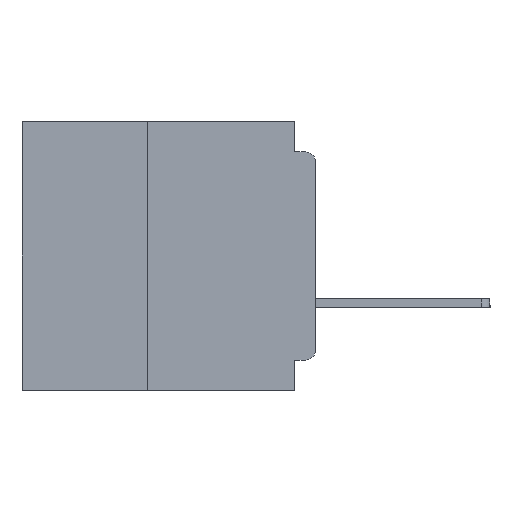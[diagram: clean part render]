
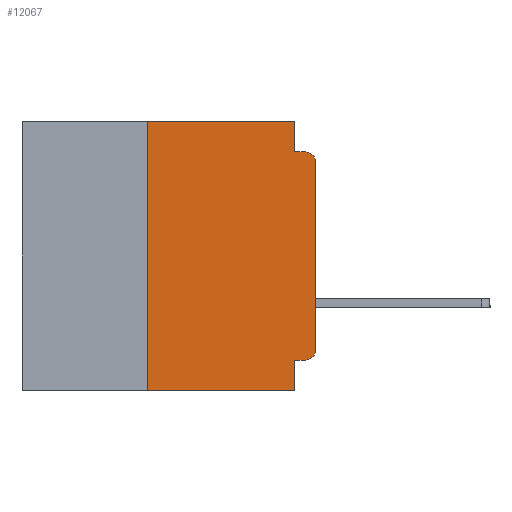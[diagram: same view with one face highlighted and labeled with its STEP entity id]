
A CAD part, left-side view. The second image highlights one B-rep face of the part: STEP entity #12067.
In plain terms, the highlighted planar face has unit normal (-1, 0, 0).
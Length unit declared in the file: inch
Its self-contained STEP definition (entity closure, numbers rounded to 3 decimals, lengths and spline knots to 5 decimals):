
#602 = ORIENTED_EDGE ( 'NONE', *, *, #23566, .F. ) ;
#1863 = DIRECTION ( 'NONE',  ( 0., 0., -1. ) ) ;
#2235 = CARTESIAN_POINT ( 'NONE',  ( 0., 0.25, -0.4 ) ) ;
#2286 = AXIS2_PLACEMENT_3D ( 'NONE', #53753, #27818, #1863 ) ;
#2663 = VECTOR ( 'NONE', #52290, 39.37008 ) ;
#3346 = VECTOR ( 'NONE', #3826, 39.37008 ) ;
#3826 = DIRECTION ( 'NONE',  ( 0., 0., -1. ) ) ;
#4662 = VECTOR ( 'NONE', #11409, 39.37008 ) ;
#4907 = CARTESIAN_POINT ( 'NONE',  ( 0., 0.031, 0. ) ) ;
#6479 = ORIENTED_EDGE ( 'NONE', *, *, #24296, .T. ) ;
#6592 = EDGE_CURVE ( 'NONE', #40797, #20047, #38859, .T. ) ;
#7959 = LINE ( 'NONE', #48586, #51354 ) ;
#8475 = VERTEX_POINT ( 'NONE', #20913 ) ;
#8895 = EDGE_LOOP ( 'NONE', ( #35240, #6479, #44124, #34297, #18049, #14018, #14569, #22161, #602, #51698 ) ) ;
#9967 = VECTOR ( 'NONE', #12778, 39.37008 ) ;
#11114 = CARTESIAN_POINT ( 'NONE',  ( 0., 0.437, -0.4 ) ) ;
#11409 = DIRECTION ( 'NONE',  ( 0., 0., 1. ) ) ;
#12067 = ADVANCED_FACE ( 'NONE', ( #36100 ), #45964, .F. ) ;
#12778 = DIRECTION ( 'NONE',  ( 0., -1., 0. ) ) ;
#13039 = AXIS2_PLACEMENT_3D ( 'NONE', #48051, #22104, #52382 ) ;
#13669 = CARTESIAN_POINT ( 'NONE',  ( 0., 0.015, -0.045 ) ) ;
#14018 = ORIENTED_EDGE ( 'NONE', *, *, #47870, .F. ) ;
#14569 = ORIENTED_EDGE ( 'NONE', *, *, #6592, .T. ) ;
#15309 = CARTESIAN_POINT ( 'NONE',  ( 0., 0.031, -0.355 ) ) ;
#15488 = CARTESIAN_POINT ( 'NONE',  ( 0., 0.437, 0. ) ) ;
#15780 = EDGE_CURVE ( 'NONE', #51715, #33872, #22848, .T. ) ;
#16420 = VERTEX_POINT ( 'NONE', #36734 ) ;
#18049 = ORIENTED_EDGE ( 'NONE', *, *, #15780, .F. ) ;
#18301 = DIRECTION ( 'NONE',  ( 0., 1., 0. ) ) ;
#18519 = CIRCLE ( 'NONE', #13039, 0.015 ) ;
#19192 = EDGE_CURVE ( 'NONE', #26292, #16420, #18519, .T. ) ;
#20047 = VERTEX_POINT ( 'NONE', #54924 ) ;
#20336 = VERTEX_POINT ( 'NONE', #13669 ) ;
#20913 = CARTESIAN_POINT ( 'NONE',  ( 0., 0., -0.06 ) ) ;
#20924 = LINE ( 'NONE', #45200, #28352 ) ;
#21399 = EDGE_CURVE ( 'NONE', #50193, #20047, #46755, .T. ) ;
#22011 = CARTESIAN_POINT ( 'NONE',  ( 0., 0., 0. ) ) ;
#22104 = DIRECTION ( 'NONE',  ( -1., 0., 0. ) ) ;
#22161 = ORIENTED_EDGE ( 'NONE', *, *, #21399, .F. ) ;
#22330 = CARTESIAN_POINT ( 'NONE',  ( 0., 0.25, 0. ) ) ;
#22848 = LINE ( 'NONE', #34366, #9967 ) ;
#23197 = EDGE_CURVE ( 'NONE', #38565, #20336, #20924, .T. ) ;
#23566 = EDGE_CURVE ( 'NONE', #26292, #50193, #7959, .T. ) ;
#24149 = EDGE_CURVE ( 'NONE', #33872, #38565, #43163, .T. ) ;
#24296 = EDGE_CURVE ( 'NONE', #8475, #20336, #49253, .T. ) ;
#24360 = DIRECTION ( 'NONE',  ( 0., 0., -1. ) ) ;
#26292 = VERTEX_POINT ( 'NONE', #30067 ) ;
#27818 = DIRECTION ( 'NONE',  ( -1., 0., 0. ) ) ;
#28352 = VECTOR ( 'NONE', #32142, 39.37008 ) ;
#30067 = CARTESIAN_POINT ( 'NONE',  ( 0., 0.015, -0.355 ) ) ;
#31644 = VECTOR ( 'NONE', #35263, 39.37008 ) ;
#32142 = DIRECTION ( 'NONE',  ( 0., -1., 0. ) ) ;
#32698 = DIRECTION ( 'NONE',  ( 0., -1., 0. ) ) ;
#33872 = VERTEX_POINT ( 'NONE', #38232 ) ;
#34297 = ORIENTED_EDGE ( 'NONE', *, *, #24149, .F. ) ;
#34366 = CARTESIAN_POINT ( 'NONE',  ( 0., 0.437, 0. ) ) ;
#35240 = ORIENTED_EDGE ( 'NONE', *, *, #47668, .T. ) ;
#35263 = DIRECTION ( 'NONE',  ( 0., 0., -1. ) ) ;
#36100 = FACE_OUTER_BOUND ( 'NONE', #8895, .T. ) ;
#36734 = CARTESIAN_POINT ( 'NONE',  ( 0., 0., -0.34 ) ) ;
#37354 = CARTESIAN_POINT ( 'NONE',  ( 0., 0.25, -0.4 ) ) ;
#37524 = VECTOR ( 'NONE', #32698, 39.37008 ) ;
#38232 = CARTESIAN_POINT ( 'NONE',  ( 0., 0.031, 0. ) ) ;
#38565 = VERTEX_POINT ( 'NONE', #42870 ) ;
#38859 = LINE ( 'NONE', #11114, #37524 ) ;
#40007 = AXIS2_PLACEMENT_3D ( 'NONE', #15488, #50309, #24360 ) ;
#40797 = VERTEX_POINT ( 'NONE', #2235 ) ;
#41995 = LINE ( 'NONE', #37354, #4662 ) ;
#42870 = CARTESIAN_POINT ( 'NONE',  ( 0., 0.031, -0.045 ) ) ;
#43163 = LINE ( 'NONE', #4907, #31644 ) ;
#44124 = ORIENTED_EDGE ( 'NONE', *, *, #23197, .F. ) ;
#45200 = CARTESIAN_POINT ( 'NONE',  ( 0., 0., -0.045 ) ) ;
#45964 = PLANE ( 'NONE',  #40007 ) ;
#46755 = LINE ( 'NONE', #51044, #3346 ) ;
#47668 = EDGE_CURVE ( 'NONE', #16420, #8475, #48799, .T. ) ;
#47870 = EDGE_CURVE ( 'NONE', #40797, #51715, #41995, .T. ) ;
#48051 = CARTESIAN_POINT ( 'NONE',  ( 0., 0.015, -0.34 ) ) ;
#48586 = CARTESIAN_POINT ( 'NONE',  ( 0., 0., -0.355 ) ) ;
#48799 = LINE ( 'NONE', #22011, #2663 ) ;
#49253 = CIRCLE ( 'NONE', #2286, 0.015 ) ;
#50193 = VERTEX_POINT ( 'NONE', #15309 ) ;
#50309 = DIRECTION ( 'NONE',  ( 1., 0., 0. ) ) ;
#51044 = CARTESIAN_POINT ( 'NONE',  ( 0., 0.031, -0.4 ) ) ;
#51354 = VECTOR ( 'NONE', #18301, 39.37008 ) ;
#51698 = ORIENTED_EDGE ( 'NONE', *, *, #19192, .T. ) ;
#51715 = VERTEX_POINT ( 'NONE', #22330 ) ;
#52290 = DIRECTION ( 'NONE',  ( 0., 0., 1. ) ) ;
#52382 = DIRECTION ( 'NONE',  ( 0., 0., -1. ) ) ;
#53753 = CARTESIAN_POINT ( 'NONE',  ( 0., 0.015, -0.06 ) ) ;
#54924 = CARTESIAN_POINT ( 'NONE',  ( 0., 0.031, -0.4 ) ) ;
